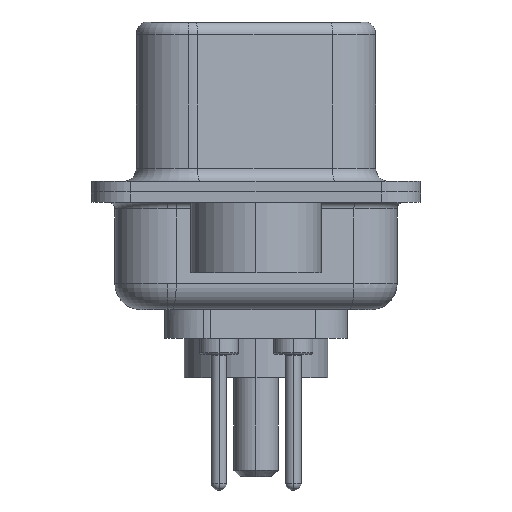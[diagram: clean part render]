
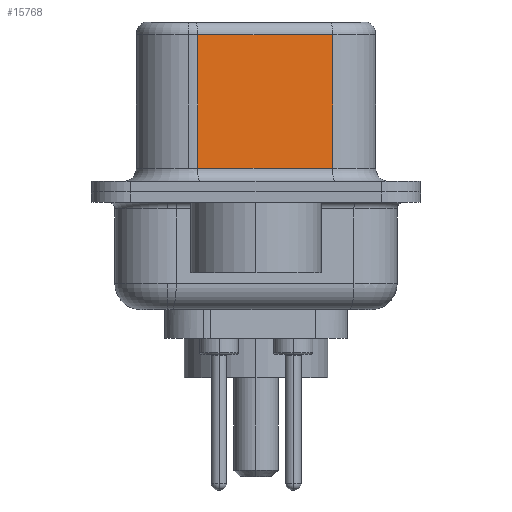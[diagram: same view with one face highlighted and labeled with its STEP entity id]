
A CAD part, left-side view. The second image highlights one B-rep face of the part: STEP entity #15768.
In plain terms, the highlighted planar face has unit normal (-0.985, -0.174, 0).
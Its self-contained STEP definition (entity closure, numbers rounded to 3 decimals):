
#135 = DIRECTION ( 'NONE',  ( 0., 0., -1. ) ) ;
#528 = CARTESIAN_POINT ( 'NONE',  ( 3.67, 2.233, 0.9 ) ) ;
#538 = DIRECTION ( 'NONE',  ( 0., 0., -1. ) ) ;
#750 = PLANE ( 'NONE',  #13431 ) ;
#1545 = LINE ( 'NONE', #5998, #11569 ) ;
#1881 = CARTESIAN_POINT ( 'NONE',  ( 4.58, -2.927, 0.9 ) ) ;
#3066 = CARTESIAN_POINT ( 'NONE',  ( 4.58, -2.927, 6.02 ) ) ;
#3244 = ORIENTED_EDGE ( 'NONE', *, *, #10046, .T. ) ;
#3504 = LINE ( 'NONE', #8402, #16796 ) ;
#3638 = VERTEX_POINT ( 'NONE', #8109 ) ;
#4285 = ORIENTED_EDGE ( 'NONE', *, *, #6089, .F. ) ;
#4653 = ORIENTED_EDGE ( 'NONE', *, *, #8104, .T. ) ;
#5778 = EDGE_CURVE ( 'NONE', #15696, #9367, #12185, .T. ) ;
#5998 = CARTESIAN_POINT ( 'NONE',  ( 4.58, -2.927, 6.52 ) ) ;
#6024 = CARTESIAN_POINT ( 'NONE',  ( 4.58, -2.927, 6.52 ) ) ;
#6089 = EDGE_CURVE ( 'NONE', #3638, #9367, #1545, .T. ) ;
#7317 = CARTESIAN_POINT ( 'NONE',  ( 3.67, 2.233, 6.02 ) ) ;
#7350 = DIRECTION ( 'NONE',  ( -0.174, 0.985, 0. ) ) ;
#7516 = VERTEX_POINT ( 'NONE', #7317 ) ;
#8104 = EDGE_CURVE ( 'NONE', #3638, #7516, #12156, .T. ) ;
#8109 = CARTESIAN_POINT ( 'NONE',  ( 4.58, -2.927, 6.02 ) ) ;
#8402 = CARTESIAN_POINT ( 'NONE',  ( 3.67, 2.233, 6.52 ) ) ;
#8711 = ORIENTED_EDGE ( 'NONE', *, *, #5778, .T. ) ;
#8981 = DIRECTION ( 'NONE',  ( 0.174, -0.985, 0. ) ) ;
#9367 = VERTEX_POINT ( 'NONE', #13306 ) ;
#9870 = EDGE_LOOP ( 'NONE', ( #4285, #4653, #3244, #8711 ) ) ;
#10046 = EDGE_CURVE ( 'NONE', #7516, #15696, #3504, .T. ) ;
#10729 = DIRECTION ( 'NONE',  ( -0.174, 0.985, 0. ) ) ;
#11569 = VECTOR ( 'NONE', #135, 1000. ) ;
#12156 = LINE ( 'NONE', #3066, #14690 ) ;
#12185 = LINE ( 'NONE', #1881, #15084 ) ;
#13306 = CARTESIAN_POINT ( 'NONE',  ( 4.58, -2.927, 0.9 ) ) ;
#13431 = AXIS2_PLACEMENT_3D ( 'NONE', #6024, #15030, #7350 ) ;
#13685 = FACE_OUTER_BOUND ( 'NONE', #9870, .T. ) ;
#14690 = VECTOR ( 'NONE', #10729, 1000. ) ;
#15030 = DIRECTION ( 'NONE',  ( 0.985, 0.174, 0. ) ) ;
#15084 = VECTOR ( 'NONE', #8981, 1000. ) ;
#15696 = VERTEX_POINT ( 'NONE', #528 ) ;
#15768 = ADVANCED_FACE ( 'NONE', ( #13685 ), #750, .F. ) ;
#16796 = VECTOR ( 'NONE', #538, 1000. ) ;
